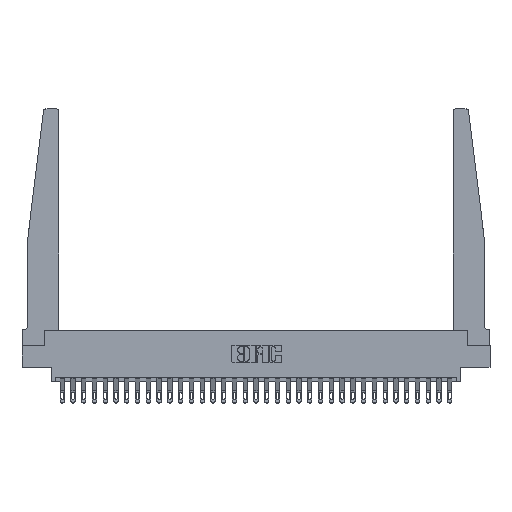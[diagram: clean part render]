
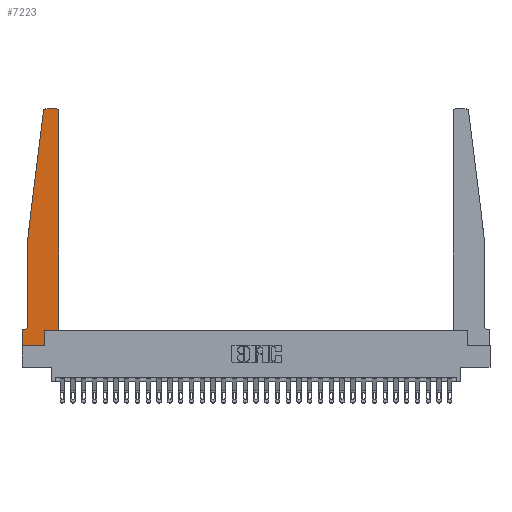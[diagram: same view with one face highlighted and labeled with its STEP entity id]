
A CAD part, top view. The second image highlights one B-rep face of the part: STEP entity #7223.
In plain terms, the highlighted planar face has unit normal (0, 0, 1).
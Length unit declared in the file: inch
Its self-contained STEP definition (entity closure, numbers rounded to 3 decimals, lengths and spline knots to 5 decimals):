
#65 = CARTESIAN_POINT ( 'NONE',  ( 0.395, 2.75, 0.37 ) ) ;
#903 = VECTOR ( 'NONE', #8293, 39.37008 ) ;
#1017 = VERTEX_POINT ( 'NONE', #26085 ) ;
#1655 = DIRECTION ( 'NONE',  ( 0., 0., 1. ) ) ;
#1934 = DIRECTION ( 'NONE',  ( 0., 0., -1. ) ) ;
#2154 = EDGE_CURVE ( 'NONE', #3777, #1017, #11574, .T. ) ;
#2267 = LINE ( 'NONE', #19700, #6277 ) ;
#2420 = CARTESIAN_POINT ( 'NONE',  ( 0.065, 0.2375, 0.37 ) ) ;
#2494 = VERTEX_POINT ( 'NONE', #17937 ) ;
#2510 = CARTESIAN_POINT ( 'NONE',  ( 0.065, 0.1875, 0.37 ) ) ;
#2530 = DIRECTION ( 'NONE',  ( 0., -1., 0. ) ) ;
#2664 = VERTEX_POINT ( 'NONE', #22687 ) ;
#3566 = DIRECTION ( 'NONE',  ( 1., 0., 0. ) ) ;
#3777 = VERTEX_POINT ( 'NONE', #29541 ) ;
#3883 = VERTEX_POINT ( 'NONE', #11697 ) ;
#3933 = EDGE_CURVE ( 'NONE', #2494, #17584, #24147, .T. ) ;
#4591 = VERTEX_POINT ( 'NONE', #65 ) ;
#4867 = DIRECTION ( 'NONE',  ( -1., 0., 0. ) ) ;
#4896 = ORIENTED_EDGE ( 'NONE', *, *, #12440, .T. ) ;
#5064 = EDGE_CURVE ( 'NONE', #3883, #3777, #23462, .T. ) ;
#5496 = LINE ( 'NONE', #21125, #11693 ) ;
#5693 = EDGE_CURVE ( 'NONE', #26521, #12171, #12927, .T. ) ;
#5812 = DIRECTION ( 'NONE',  ( 0., -1., 0. ) ) ;
#6277 = VECTOR ( 'NONE', #22044, 39.37008 ) ;
#6717 = VECTOR ( 'NONE', #27523, 39.37008 ) ;
#7223 = ADVANCED_FACE ( 'NONE', ( #18062 ), #26719, .T. ) ;
#7284 = VERTEX_POINT ( 'NONE', #10123 ) ;
#7474 = CARTESIAN_POINT ( 'NONE',  ( 0.065, 1.25, 0.37 ) ) ;
#7763 = VECTOR ( 'NONE', #23597, 39.37008 ) ;
#7803 = ORIENTED_EDGE ( 'NONE', *, *, #26112, .T. ) ;
#7944 = CARTESIAN_POINT ( 'NONE',  ( 0.065, 1.25, 0.37 ) ) ;
#8106 = ORIENTED_EDGE ( 'NONE', *, *, #2154, .T. ) ;
#8293 = DIRECTION ( 'NONE',  ( 1., 0., 0. ) ) ;
#8711 = DIRECTION ( 'NONE',  ( 0., 1., 0. ) ) ;
#8975 = CARTESIAN_POINT ( 'NONE',  ( 0., 0., 0.37 ) ) ;
#9848 = DIRECTION ( 'NONE',  ( -0.122, -0.992, 0. ) ) ;
#9883 = EDGE_LOOP ( 'NONE', ( #19467, #21130, #8106, #25036, #25937, #12552, #4896, #13800, #28336, #10908, #14546, #7803 ) ) ;
#10087 = VERTEX_POINT ( 'NONE', #2420 ) ;
#10123 = CARTESIAN_POINT ( 'NONE',  ( 0.425, 0.18, 0.37 ) ) ;
#10281 = CARTESIAN_POINT ( 'NONE',  ( 0.2605, 0., 0.37 ) ) ;
#10908 = ORIENTED_EDGE ( 'NONE', *, *, #25292, .T. ) ;
#11574 = LINE ( 'NONE', #7474, #26224 ) ;
#11693 = VECTOR ( 'NONE', #2530, 39.37008 ) ;
#11697 = CARTESIAN_POINT ( 'NONE',  ( 0.27653, 2.75, 0.37 ) ) ;
#12171 = VERTEX_POINT ( 'NONE', #10281 ) ;
#12234 = CARTESIAN_POINT ( 'NONE',  ( 0.2605, 0.18, 0.37 ) ) ;
#12440 = EDGE_CURVE ( 'NONE', #17584, #26521, #5496, .T. ) ;
#12552 = ORIENTED_EDGE ( 'NONE', *, *, #3933, .T. ) ;
#12615 = VECTOR ( 'NONE', #5812, 39.37008 ) ;
#12842 = CARTESIAN_POINT ( 'NONE',  ( 0., 0.1875, 0.37 ) ) ;
#12927 = LINE ( 'NONE', #8975, #6717 ) ;
#13731 = DIRECTION ( 'NONE',  ( 0., 0., 1. ) ) ;
#13800 = ORIENTED_EDGE ( 'NONE', *, *, #5693, .T. ) ;
#14546 = ORIENTED_EDGE ( 'NONE', *, *, #19600, .T. ) ;
#14968 = AXIS2_PLACEMENT_3D ( 'NONE', #12842, #17501, #3566 ) ;
#15283 = CARTESIAN_POINT ( 'NONE',  ( 0.425, 0.18, 0.37 ) ) ;
#15581 = CARTESIAN_POINT ( 'NONE',  ( 0.27653, 2.72, 0.37 ) ) ;
#15608 = EDGE_CURVE ( 'NONE', #10087, #2494, #27452, .T. ) ;
#15864 = CARTESIAN_POINT ( 'NONE',  ( 0.015, 0.2375, 0.37 ) ) ;
#17501 = DIRECTION ( 'NONE',  ( 0., 0., 1. ) ) ;
#17584 = VERTEX_POINT ( 'NONE', #23059 ) ;
#17626 = AXIS2_PLACEMENT_3D ( 'NONE', #15864, #1934, #18211 ) ;
#17928 = DIRECTION ( 'NONE',  ( 1., 0., 0. ) ) ;
#17933 = EDGE_CURVE ( 'NONE', #12171, #27184, #2267, .T. ) ;
#17937 = CARTESIAN_POINT ( 'NONE',  ( 0.015, 0.1875, 0.37 ) ) ;
#17998 = LINE ( 'NONE', #15283, #903 ) ;
#18062 = FACE_OUTER_BOUND ( 'NONE', #9883, .T. ) ;
#18187 = LINE ( 'NONE', #27159, #23595 ) ;
#18211 = DIRECTION ( 'NONE',  ( -1., 0., 0. ) ) ;
#18787 = LINE ( 'NONE', #7944, #12615 ) ;
#19057 = CARTESIAN_POINT ( 'NONE',  ( 0.25, 2.75, 0.37 ) ) ;
#19467 = ORIENTED_EDGE ( 'NONE', *, *, #24020, .T. ) ;
#19482 = CARTESIAN_POINT ( 'NONE',  ( 0., 0., 0.37 ) ) ;
#19600 = EDGE_CURVE ( 'NONE', #7284, #2664, #18187, .T. ) ;
#19700 = CARTESIAN_POINT ( 'NONE',  ( 0.2605, 0.18, 0.37 ) ) ;
#21125 = CARTESIAN_POINT ( 'NONE',  ( 0., 0., 0.37 ) ) ;
#21130 = ORIENTED_EDGE ( 'NONE', *, *, #5064, .T. ) ;
#21188 = EDGE_CURVE ( 'NONE', #1017, #10087, #18787, .T. ) ;
#21559 = CIRCLE ( 'NONE', #24596, 0.03 ) ;
#21990 = VECTOR ( 'NONE', #4867, 39.37008 ) ;
#22044 = DIRECTION ( 'NONE',  ( 0., 1., 0. ) ) ;
#22687 = CARTESIAN_POINT ( 'NONE',  ( 0.425, 2.72, 0.37 ) ) ;
#23059 = CARTESIAN_POINT ( 'NONE',  ( 0., 0.1875, 0.37 ) ) ;
#23462 = CIRCLE ( 'NONE', #28417, 0.03 ) ;
#23595 = VECTOR ( 'NONE', #8711, 39.37008 ) ;
#23597 = DIRECTION ( 'NONE',  ( -1., 0., 0. ) ) ;
#24020 = EDGE_CURVE ( 'NONE', #4591, #3883, #24834, .T. ) ;
#24147 = LINE ( 'NONE', #2510, #21990 ) ;
#24596 = AXIS2_PLACEMENT_3D ( 'NONE', #27620, #13731, #29950 ) ;
#24834 = LINE ( 'NONE', #19057, #7763 ) ;
#25036 = ORIENTED_EDGE ( 'NONE', *, *, #21188, .T. ) ;
#25292 = EDGE_CURVE ( 'NONE', #27184, #7284, #17998, .T. ) ;
#25937 = ORIENTED_EDGE ( 'NONE', *, *, #15608, .T. ) ;
#26085 = CARTESIAN_POINT ( 'NONE',  ( 0.065, 1.25, 0.37 ) ) ;
#26112 = EDGE_CURVE ( 'NONE', #2664, #4591, #21559, .T. ) ;
#26224 = VECTOR ( 'NONE', #9848, 39.37008 ) ;
#26521 = VERTEX_POINT ( 'NONE', #19482 ) ;
#26719 = PLANE ( 'NONE',  #14968 ) ;
#27159 = CARTESIAN_POINT ( 'NONE',  ( 0.425, 0.18, 0.37 ) ) ;
#27184 = VERTEX_POINT ( 'NONE', #12234 ) ;
#27452 = CIRCLE ( 'NONE', #17626, 0.05 ) ;
#27523 = DIRECTION ( 'NONE',  ( 1., 0., 0. ) ) ;
#27620 = CARTESIAN_POINT ( 'NONE',  ( 0.395, 2.72, 0.37 ) ) ;
#28336 = ORIENTED_EDGE ( 'NONE', *, *, #17933, .T. ) ;
#28417 = AXIS2_PLACEMENT_3D ( 'NONE', #15581, #1655, #17928 ) ;
#29541 = CARTESIAN_POINT ( 'NONE',  ( 0.24675, 2.72367, 0.37 ) ) ;
#29950 = DIRECTION ( 'NONE',  ( 1., 0., 0. ) ) ;
